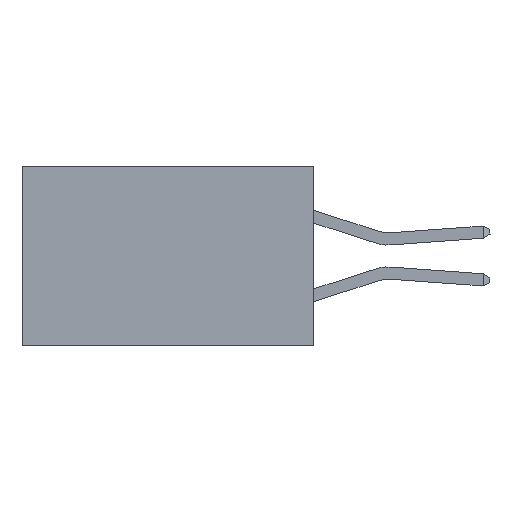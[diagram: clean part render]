
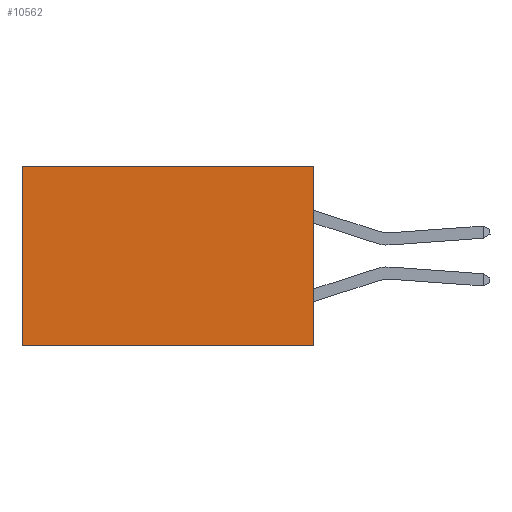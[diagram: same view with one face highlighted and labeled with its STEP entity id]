
A CAD part, left-side view. The second image highlights one B-rep face of the part: STEP entity #10562.
In plain terms, the highlighted planar face has unit normal (-1, 0, 0).
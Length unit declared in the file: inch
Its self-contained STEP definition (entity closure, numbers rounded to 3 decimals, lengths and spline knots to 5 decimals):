
#18 = DIRECTION ( 'NONE',  ( 0., 1., 0. ) ) ;
#726 = VECTOR ( 'NONE', #11072, 39.37008 ) ;
#832 = LINE ( 'NONE', #14754, #5630 ) ;
#854 = CARTESIAN_POINT ( 'NONE',  ( 0.2875, 0., 0. ) ) ;
#1257 = CARTESIAN_POINT ( 'NONE',  ( 0.2875, 0.6, -0.37 ) ) ;
#1698 = DIRECTION ( 'NONE',  ( 0., 0., -1. ) ) ;
#1761 = LINE ( 'NONE', #10957, #726 ) ;
#2591 = EDGE_CURVE ( 'NONE', #7385, #5357, #832, .T. ) ;
#3117 = PLANE ( 'NONE',  #3784 ) ;
#3146 = CARTESIAN_POINT ( 'NONE',  ( 0.2875, 0., 0. ) ) ;
#3593 = DIRECTION ( 'NONE',  ( 0., 0., -1. ) ) ;
#3752 = VECTOR ( 'NONE', #18, 39.37008 ) ;
#3784 = AXIS2_PLACEMENT_3D ( 'NONE', #13775, #5817, #1698 ) ;
#3985 = CARTESIAN_POINT ( 'NONE',  ( 0.2875, 0., 0. ) ) ;
#4274 = EDGE_CURVE ( 'NONE', #5173, #7385, #14343, .T. ) ;
#5173 = VERTEX_POINT ( 'NONE', #3146 ) ;
#5357 = VERTEX_POINT ( 'NONE', #1257 ) ;
#5449 = CARTESIAN_POINT ( 'NONE',  ( 0.2875, 0.6, 0. ) ) ;
#5630 = VECTOR ( 'NONE', #5636, 39.37008 ) ;
#5636 = DIRECTION ( 'NONE',  ( 0., 1., 0. ) ) ;
#5817 = DIRECTION ( 'NONE',  ( 1., 0., 0. ) ) ;
#7385 = VERTEX_POINT ( 'NONE', #14534 ) ;
#7482 = VERTEX_POINT ( 'NONE', #5449 ) ;
#7630 = ORIENTED_EDGE ( 'NONE', *, *, #4274, .F. ) ;
#9368 = ORIENTED_EDGE ( 'NONE', *, *, #10550, .T. ) ;
#9901 = EDGE_CURVE ( 'NONE', #5173, #7482, #13107, .T. ) ;
#10550 = EDGE_CURVE ( 'NONE', #7482, #5357, #1761, .T. ) ;
#10562 = ADVANCED_FACE ( 'NONE', ( #14464 ), #3117, .F. ) ;
#10957 = CARTESIAN_POINT ( 'NONE',  ( 0.2875, 0.6, 0. ) ) ;
#11072 = DIRECTION ( 'NONE',  ( 0., 0., -1. ) ) ;
#12035 = VECTOR ( 'NONE', #3593, 39.37008 ) ;
#13107 = LINE ( 'NONE', #3985, #3752 ) ;
#13775 = CARTESIAN_POINT ( 'NONE',  ( 0.2875, 0., 0. ) ) ;
#14343 = LINE ( 'NONE', #854, #12035 ) ;
#14464 = FACE_OUTER_BOUND ( 'NONE', #14915, .T. ) ;
#14534 = CARTESIAN_POINT ( 'NONE',  ( 0.2875, 0., -0.37 ) ) ;
#14754 = CARTESIAN_POINT ( 'NONE',  ( 0.2875, 0., -0.37 ) ) ;
#14915 = EDGE_LOOP ( 'NONE', ( #9368, #16858, #7630, #16705 ) ) ;
#16705 = ORIENTED_EDGE ( 'NONE', *, *, #9901, .T. ) ;
#16858 = ORIENTED_EDGE ( 'NONE', *, *, #2591, .F. ) ;
